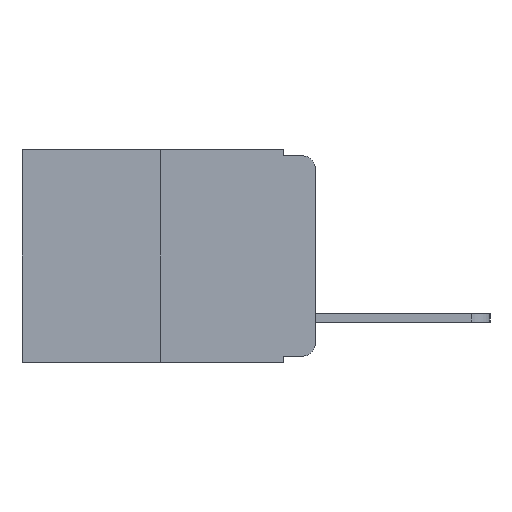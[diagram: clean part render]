
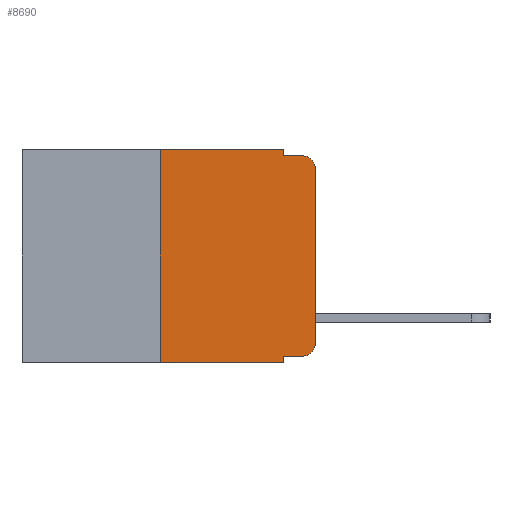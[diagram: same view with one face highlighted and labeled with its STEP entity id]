
A CAD part, left-side view. The second image highlights one B-rep face of the part: STEP entity #8690.
In plain terms, the highlighted planar face has unit normal (-1, 0, 0).
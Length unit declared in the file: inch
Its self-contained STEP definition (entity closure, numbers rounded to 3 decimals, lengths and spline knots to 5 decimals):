
#343 = LINE ( 'NONE', #9479, #6515 ) ;
#602 = ORIENTED_EDGE ( 'NONE', *, *, #5079, .F. ) ;
#758 = PLANE ( 'NONE',  #14256 ) ;
#1319 = VECTOR ( 'NONE', #3222, 39.37008 ) ;
#1335 = DIRECTION ( 'NONE',  ( 0., 0., -1. ) ) ;
#1512 = ORIENTED_EDGE ( 'NONE', *, *, #1813, .F. ) ;
#1706 = DIRECTION ( 'NONE',  ( -1., 0., 0. ) ) ;
#1764 = EDGE_CURVE ( 'NONE', #4106, #12024, #10195, .T. ) ;
#1813 = EDGE_CURVE ( 'NONE', #4106, #7209, #343, .T. ) ;
#2156 = DIRECTION ( 'NONE',  ( 0., 0., -1. ) ) ;
#2529 = VERTEX_POINT ( 'NONE', #11621 ) ;
#2535 = CIRCLE ( 'NONE', #2915, 0.02 ) ;
#2756 = DIRECTION ( 'NONE',  ( 0., 0., 1. ) ) ;
#2778 = VERTEX_POINT ( 'NONE', #14295 ) ;
#2915 = AXIS2_PLACEMENT_3D ( 'NONE', #10949, #4042, #11989 ) ;
#3200 = LINE ( 'NONE', #8627, #14652 ) ;
#3201 = CARTESIAN_POINT ( 'NONE',  ( 0., 0.25, -0.343 ) ) ;
#3222 = DIRECTION ( 'NONE',  ( 0., -1., 0. ) ) ;
#4029 = VECTOR ( 'NONE', #12803, 39.37008 ) ;
#4042 = DIRECTION ( 'NONE',  ( -1., 0., 0. ) ) ;
#4106 = VERTEX_POINT ( 'NONE', #12961 ) ;
#4125 = EDGE_CURVE ( 'NONE', #7563, #13783, #9808, .T. ) ;
#4270 = ORIENTED_EDGE ( 'NONE', *, *, #5929, .F. ) ;
#4590 = EDGE_CURVE ( 'NONE', #4872, #2529, #5152, .T. ) ;
#4813 = CARTESIAN_POINT ( 'NONE',  ( 0., 0.02, -0.333 ) ) ;
#4872 = VERTEX_POINT ( 'NONE', #12606 ) ;
#4884 = AXIS2_PLACEMENT_3D ( 'NONE', #9036, #1706, #10144 ) ;
#5071 = ORIENTED_EDGE ( 'NONE', *, *, #1764, .T. ) ;
#5079 = EDGE_CURVE ( 'NONE', #10852, #4872, #8081, .T. ) ;
#5152 = LINE ( 'NONE', #8030, #10820 ) ;
#5711 = EDGE_LOOP ( 'NONE', ( #9692, #12465, #12848, #602, #4270, #13141, #7847, #1512, #5071, #8180 ) ) ;
#5738 = CARTESIAN_POINT ( 'NONE',  ( 0., 0.473, 0. ) ) ;
#5929 = EDGE_CURVE ( 'NONE', #13783, #10852, #11258, .T. ) ;
#5989 = CIRCLE ( 'NONE', #4884, 0.02 ) ;
#6057 = CARTESIAN_POINT ( 'NONE',  ( 0., 0.051, 0. ) ) ;
#6515 = VECTOR ( 'NONE', #13028, 39.37008 ) ;
#6520 = EDGE_CURVE ( 'NONE', #7563, #7209, #3200, .T. ) ;
#6533 = CARTESIAN_POINT ( 'NONE',  ( 0., 0.051, 0. ) ) ;
#6681 = EDGE_CURVE ( 'NONE', #14672, #2529, #5989, .T. ) ;
#6711 = EDGE_CURVE ( 'NONE', #2778, #14672, #14189, .T. ) ;
#7209 = VERTEX_POINT ( 'NONE', #13080 ) ;
#7563 = VERTEX_POINT ( 'NONE', #3201 ) ;
#7847 = ORIENTED_EDGE ( 'NONE', *, *, #6520, .T. ) ;
#8030 = CARTESIAN_POINT ( 'NONE',  ( 0., 0.051, -0.01 ) ) ;
#8051 = CARTESIAN_POINT ( 'NONE',  ( 0., 0.25, 0. ) ) ;
#8081 = LINE ( 'NONE', #6533, #13356 ) ;
#8180 = ORIENTED_EDGE ( 'NONE', *, *, #10117, .T. ) ;
#8317 = VECTOR ( 'NONE', #10196, 39.37008 ) ;
#8627 = CARTESIAN_POINT ( 'NONE',  ( 0., 0.473, -0.343 ) ) ;
#8690 = ADVANCED_FACE ( 'NONE', ( #9507 ), #758, .F. ) ;
#9036 = CARTESIAN_POINT ( 'NONE',  ( 0., 0.02, -0.03 ) ) ;
#9082 = CARTESIAN_POINT ( 'NONE',  ( 0., 0., 0. ) ) ;
#9417 = DIRECTION ( 'NONE',  ( 1., 0., 0. ) ) ;
#9479 = CARTESIAN_POINT ( 'NONE',  ( 0., 0.051, 0. ) ) ;
#9507 = FACE_OUTER_BOUND ( 'NONE', #5711, .T. ) ;
#9692 = ORIENTED_EDGE ( 'NONE', *, *, #6711, .T. ) ;
#9808 = LINE ( 'NONE', #14939, #11988 ) ;
#10117 = EDGE_CURVE ( 'NONE', #12024, #2778, #2535, .T. ) ;
#10144 = DIRECTION ( 'NONE',  ( 0., 0., -1. ) ) ;
#10195 = LINE ( 'NONE', #12707, #4029 ) ;
#10196 = DIRECTION ( 'NONE',  ( 0., 0., 1. ) ) ;
#10820 = VECTOR ( 'NONE', #14265, 39.37008 ) ;
#10852 = VERTEX_POINT ( 'NONE', #6057 ) ;
#10949 = CARTESIAN_POINT ( 'NONE',  ( 0., 0.02, -0.313 ) ) ;
#11258 = LINE ( 'NONE', #5738, #1319 ) ;
#11265 = CARTESIAN_POINT ( 'NONE',  ( 0., 0., -0.03 ) ) ;
#11621 = CARTESIAN_POINT ( 'NONE',  ( 0., 0.02, -0.01 ) ) ;
#11988 = VECTOR ( 'NONE', #2756, 39.37008 ) ;
#11989 = DIRECTION ( 'NONE',  ( 0., 0., -1. ) ) ;
#12024 = VERTEX_POINT ( 'NONE', #4813 ) ;
#12465 = ORIENTED_EDGE ( 'NONE', *, *, #6681, .T. ) ;
#12606 = CARTESIAN_POINT ( 'NONE',  ( 0., 0.051, -0.01 ) ) ;
#12707 = CARTESIAN_POINT ( 'NONE',  ( 0., 0.051, -0.333 ) ) ;
#12803 = DIRECTION ( 'NONE',  ( 0., -1., 0. ) ) ;
#12848 = ORIENTED_EDGE ( 'NONE', *, *, #4590, .F. ) ;
#12905 = DIRECTION ( 'NONE',  ( 0., -1., 0. ) ) ;
#12961 = CARTESIAN_POINT ( 'NONE',  ( 0., 0.051, -0.333 ) ) ;
#13028 = DIRECTION ( 'NONE',  ( 0., 0., -1. ) ) ;
#13080 = CARTESIAN_POINT ( 'NONE',  ( 0., 0.051, -0.343 ) ) ;
#13141 = ORIENTED_EDGE ( 'NONE', *, *, #4125, .F. ) ;
#13356 = VECTOR ( 'NONE', #1335, 39.37008 ) ;
#13559 = CARTESIAN_POINT ( 'NONE',  ( 0., 0.473, 0. ) ) ;
#13783 = VERTEX_POINT ( 'NONE', #8051 ) ;
#14189 = LINE ( 'NONE', #9082, #8317 ) ;
#14256 = AXIS2_PLACEMENT_3D ( 'NONE', #13559, #9417, #2156 ) ;
#14265 = DIRECTION ( 'NONE',  ( 0., -1., 0. ) ) ;
#14295 = CARTESIAN_POINT ( 'NONE',  ( 0., 0., -0.313 ) ) ;
#14652 = VECTOR ( 'NONE', #12905, 39.37008 ) ;
#14672 = VERTEX_POINT ( 'NONE', #11265 ) ;
#14939 = CARTESIAN_POINT ( 'NONE',  ( 0., 0.25, 0. ) ) ;
